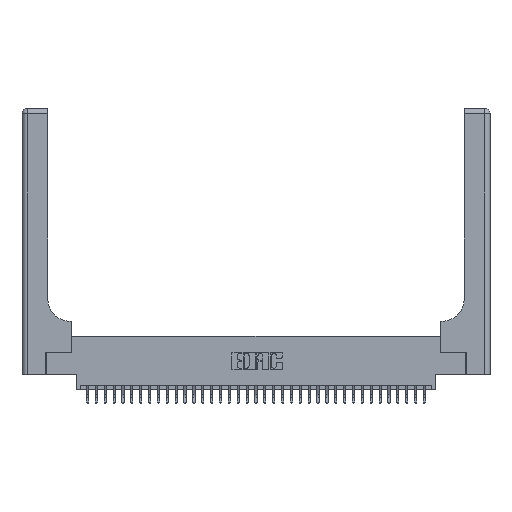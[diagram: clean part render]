
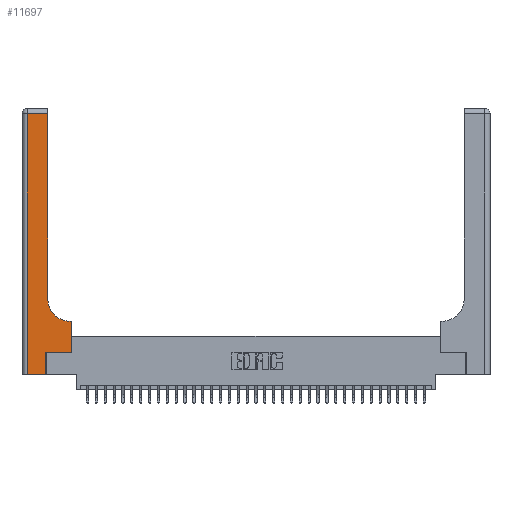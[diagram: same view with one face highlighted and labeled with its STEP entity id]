
A CAD part, top view. The second image highlights one B-rep face of the part: STEP entity #11697.
In plain terms, the highlighted planar face has unit normal (0, 0, 1).
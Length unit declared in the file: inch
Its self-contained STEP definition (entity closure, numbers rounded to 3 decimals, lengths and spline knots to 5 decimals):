
#736 = EDGE_CURVE ( 'NONE', #13942, #25288, #18136, .T. ) ;
#741 = EDGE_CURVE ( 'NONE', #10642, #3814, #4007, .T. ) ;
#998 = CARTESIAN_POINT ( 'NONE',  ( 0.5415, 0.85, 0.37 ) ) ;
#1064 = ORIENTED_EDGE ( 'NONE', *, *, #30271, .T. ) ;
#1715 = CARTESIAN_POINT ( 'NONE',  ( 0., 2.94, 0.37 ) ) ;
#2290 = LINE ( 'NONE', #29288, #35342 ) ;
#2358 = ORIENTED_EDGE ( 'NONE', *, *, #741, .T. ) ;
#3589 = DIRECTION ( 'NONE',  ( -1., 0., 0. ) ) ;
#3814 = VERTEX_POINT ( 'NONE', #4777 ) ;
#3899 = CARTESIAN_POINT ( 'NONE',  ( 0.2915, 0.85, 0.37 ) ) ;
#4007 = LINE ( 'NONE', #31182, #23419 ) ;
#4066 = CARTESIAN_POINT ( 'NONE',  ( 0.5585, 0.6, 0.37 ) ) ;
#4226 = CARTESIAN_POINT ( 'NONE',  ( 0.06, 0., 0.37 ) ) ;
#4777 = CARTESIAN_POINT ( 'NONE',  ( 0.5585, 0.25, 0.37 ) ) ;
#6188 = VERTEX_POINT ( 'NONE', #35746 ) ;
#6415 = CARTESIAN_POINT ( 'NONE',  ( 0.2915, 3., 0.37 ) ) ;
#6430 = CARTESIAN_POINT ( 'NONE',  ( 0.269, 0., 0.37 ) ) ;
#6588 = DIRECTION ( 'NONE',  ( 0., 1., 0. ) ) ;
#6913 = DIRECTION ( 'NONE',  ( 1., 0., 0. ) ) ;
#7230 = FACE_OUTER_BOUND ( 'NONE', #32777, .T. ) ;
#9218 = DIRECTION ( 'NONE',  ( 1., 0., 0. ) ) ;
#9233 = AXIS2_PLACEMENT_3D ( 'NONE', #18513, #12984, #21308 ) ;
#9752 = VECTOR ( 'NONE', #23566, 39.37008 ) ;
#9942 = ORIENTED_EDGE ( 'NONE', *, *, #34346, .T. ) ;
#10320 = VECTOR ( 'NONE', #13216, 39.37008 ) ;
#10642 = VERTEX_POINT ( 'NONE', #16100 ) ;
#10837 = ORIENTED_EDGE ( 'NONE', *, *, #22369, .T. ) ;
#11035 = ORIENTED_EDGE ( 'NONE', *, *, #28930, .T. ) ;
#11256 = LINE ( 'NONE', #17418, #32836 ) ;
#11697 = ADVANCED_FACE ( 'NONE', ( #7230 ), #32553, .F. ) ;
#12984 = DIRECTION ( 'NONE',  ( 0., 0., -1. ) ) ;
#13216 = DIRECTION ( 'NONE',  ( -1., 0., 0. ) ) ;
#13942 = VERTEX_POINT ( 'NONE', #3899 ) ;
#14201 = CIRCLE ( 'NONE', #29149, 0.25 ) ;
#14254 = LINE ( 'NONE', #35343, #19087 ) ;
#14958 = ORIENTED_EDGE ( 'NONE', *, *, #28475, .T. ) ;
#15780 = CARTESIAN_POINT ( 'NONE',  ( 0.2915, 2.94, 0.37 ) ) ;
#16100 = CARTESIAN_POINT ( 'NONE',  ( 0.269, 0.25, 0.37 ) ) ;
#17418 = CARTESIAN_POINT ( 'NONE',  ( 0.2915, 0.6, 0.37 ) ) ;
#18136 = LINE ( 'NONE', #6415, #9752 ) ;
#18242 = LINE ( 'NONE', #1715, #10320 ) ;
#18513 = CARTESIAN_POINT ( 'NONE',  ( 0., 3., 0.37 ) ) ;
#19087 = VECTOR ( 'NONE', #26708, 39.37008 ) ;
#20737 = DIRECTION ( 'NONE',  ( 0., 0., -1. ) ) ;
#21308 = DIRECTION ( 'NONE',  ( -1., 0., 0. ) ) ;
#21481 = EDGE_CURVE ( 'NONE', #24701, #29086, #11256, .T. ) ;
#21724 = DIRECTION ( 'NONE',  ( 0., 1., 0. ) ) ;
#22369 = EDGE_CURVE ( 'NONE', #6188, #23102, #14254, .T. ) ;
#23102 = VERTEX_POINT ( 'NONE', #4226 ) ;
#23419 = VECTOR ( 'NONE', #6913, 39.37008 ) ;
#23566 = DIRECTION ( 'NONE',  ( 0., 1., 0. ) ) ;
#24345 = CARTESIAN_POINT ( 'NONE',  ( 0.5585, 0.25, 0.37 ) ) ;
#24701 = VERTEX_POINT ( 'NONE', #4066 ) ;
#25288 = VERTEX_POINT ( 'NONE', #15780 ) ;
#26708 = DIRECTION ( 'NONE',  ( 0., -1., 0. ) ) ;
#26734 = EDGE_CURVE ( 'NONE', #25288, #6188, #18242, .T. ) ;
#26981 = ORIENTED_EDGE ( 'NONE', *, *, #736, .T. ) ;
#28475 = EDGE_CURVE ( 'NONE', #31842, #10642, #2290, .T. ) ;
#28930 = EDGE_CURVE ( 'NONE', #29086, #13942, #14201, .T. ) ;
#29086 = VERTEX_POINT ( 'NONE', #32620 ) ;
#29149 = AXIS2_PLACEMENT_3D ( 'NONE', #998, #20737, #29525 ) ;
#29288 = CARTESIAN_POINT ( 'NONE',  ( 0.269, 0., 0.37 ) ) ;
#29525 = DIRECTION ( 'NONE',  ( 1., 0., 0. ) ) ;
#30046 = ORIENTED_EDGE ( 'NONE', *, *, #26734, .T. ) ;
#30130 = VECTOR ( 'NONE', #9218, 39.37008 ) ;
#30271 = EDGE_CURVE ( 'NONE', #3814, #24701, #36152, .T. ) ;
#31026 = LINE ( 'NONE', #32131, #30130 ) ;
#31182 = CARTESIAN_POINT ( 'NONE',  ( 0.269, 0.25, 0.37 ) ) ;
#31842 = VERTEX_POINT ( 'NONE', #6430 ) ;
#32131 = CARTESIAN_POINT ( 'NONE',  ( 0., 0., 0.37 ) ) ;
#32553 = PLANE ( 'NONE',  #9233 ) ;
#32620 = CARTESIAN_POINT ( 'NONE',  ( 0.5415, 0.6, 0.37 ) ) ;
#32777 = EDGE_LOOP ( 'NONE', ( #26981, #30046, #10837, #9942, #14958, #2358, #1064, #34835, #11035 ) ) ;
#32836 = VECTOR ( 'NONE', #3589, 39.37008 ) ;
#33500 = VECTOR ( 'NONE', #21724, 39.37008 ) ;
#34346 = EDGE_CURVE ( 'NONE', #23102, #31842, #31026, .T. ) ;
#34835 = ORIENTED_EDGE ( 'NONE', *, *, #21481, .T. ) ;
#35342 = VECTOR ( 'NONE', #6588, 39.37008 ) ;
#35343 = CARTESIAN_POINT ( 'NONE',  ( 0.06, 3., 0.37 ) ) ;
#35746 = CARTESIAN_POINT ( 'NONE',  ( 0.06, 2.94, 0.37 ) ) ;
#36152 = LINE ( 'NONE', #24345, #33500 ) ;
